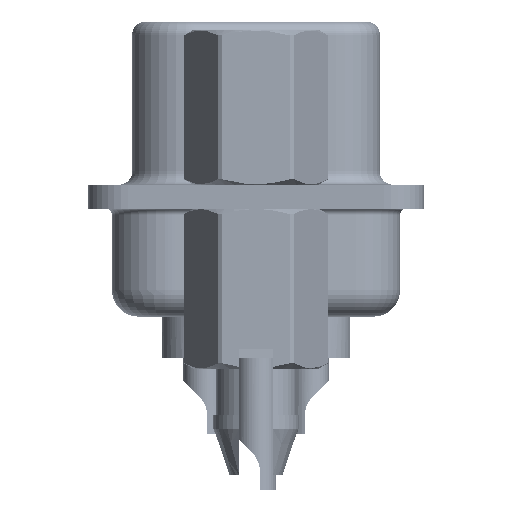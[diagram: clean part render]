
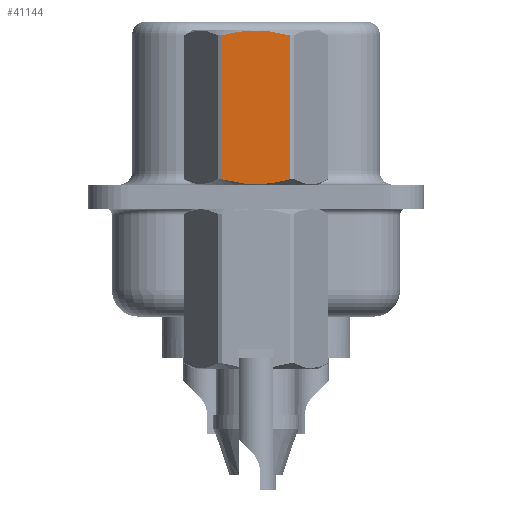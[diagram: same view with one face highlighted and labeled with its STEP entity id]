
A CAD part, left-side view. The second image highlights one B-rep face of the part: STEP entity #41144.
In plain terms, the highlighted planar face has unit normal (-1, 0, 0).
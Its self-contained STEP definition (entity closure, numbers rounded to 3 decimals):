
#478 = B_SPLINE_CURVE_WITH_KNOTS ( 'NONE', 3,
 ( #35614, #7081, #38136, #6877, #28891, #26176, #16082, #25345, #15880, #19857 ),
 .UNSPECIFIED., .F., .F.,
 ( 4, 2, 2, 2, 4 ),
 ( 0.003, 0.003, 0.004, 0.004, 0.005 ),
 .UNSPECIFIED. ) ;
#2210 = EDGE_CURVE ( 'NONE', #38166, #17996, #33887, .T. ) ;
#2494 = EDGE_CURVE ( 'NONE', #17996, #11123, #34546, .T. ) ;
#3700 = VECTOR ( 'NONE', #14819, 1000. ) ;
#4686 = DIRECTION ( 'NONE',  ( -1., 0., 0. ) ) ;
#5153 = DIRECTION ( 'NONE',  ( 0., 0., 1. ) ) ;
#6877 = CARTESIAN_POINT ( 'NONE',  ( -2.381, 0.428, 0.485 ) ) ;
#7081 = CARTESIAN_POINT ( 'NONE',  ( -2.381, 1.065, 0.596 ) ) ;
#8527 = VERTEX_POINT ( 'NONE', #16247 ) ;
#8683 = CARTESIAN_POINT ( 'NONE',  ( -2.381, -1.273, 6.048 ) ) ;
#10982 = PLANE ( 'NONE',  #33398 ) ;
#11123 = VERTEX_POINT ( 'NONE', #40946 ) ;
#12455 = CARTESIAN_POINT ( 'NONE',  ( -2.381, -1.066, 6.104 ) ) ;
#12660 = CARTESIAN_POINT ( 'NONE',  ( -2.381, -0.432, 6.215 ) ) ;
#13922 = CARTESIAN_POINT ( 'NONE',  ( -2.381, 1.375, -3.75 ) ) ;
#14133 = DIRECTION ( 'NONE',  ( 0., -1., 0. ) ) ;
#14336 = EDGE_CURVE ( 'NONE', #8527, #38166, #478, .T. ) ;
#14734 = FACE_OUTER_BOUND ( 'NONE', #26345, .T. ) ;
#14819 = DIRECTION ( 'NONE',  ( 0., 0., -1. ) ) ;
#15880 = CARTESIAN_POINT ( 'NONE',  ( -2.381, -1.066, 0.596 ) ) ;
#16082 = CARTESIAN_POINT ( 'NONE',  ( -2.381, -0.432, 0.485 ) ) ;
#16151 = VECTOR ( 'NONE', #5153, 1000. ) ;
#16247 = CARTESIAN_POINT ( 'NONE',  ( -2.381, 1.273, 0.652 ) ) ;
#17996 = VERTEX_POINT ( 'NONE', #21901 ) ;
#18160 = CARTESIAN_POINT ( 'NONE',  ( -2.381, -1.273, 3.792 ) ) ;
#19857 = CARTESIAN_POINT ( 'NONE',  ( -2.381, -1.273, 0.652 ) ) ;
#21158 = ORIENTED_EDGE ( 'NONE', *, *, #36408, .T. ) ;
#21901 = CARTESIAN_POINT ( 'NONE',  ( -2.381, -1.273, 6.048 ) ) ;
#21937 = CARTESIAN_POINT ( 'NONE',  ( -2.381, -1.273, 0.652 ) ) ;
#22112 = CARTESIAN_POINT ( 'NONE',  ( -2.381, 1.273, 6.048 ) ) ;
#23888 = LINE ( 'NONE', #24491, #3700 ) ;
#24491 = CARTESIAN_POINT ( 'NONE',  ( -2.381, 1.273, 3.792 ) ) ;
#25345 = CARTESIAN_POINT ( 'NONE',  ( -2.381, -0.858, 0.55 ) ) ;
#25475 = CARTESIAN_POINT ( 'NONE',  ( -2.381, -0.215, 6.232 ) ) ;
#26176 = CARTESIAN_POINT ( 'NONE',  ( -2.381, -0.215, 0.468 ) ) ;
#26345 = EDGE_LOOP ( 'NONE', ( #36290, #35183, #34044, #21158 ) ) ;
#28185 = CARTESIAN_POINT ( 'NONE',  ( -2.381, 0.853, 6.151 ) ) ;
#28610 = CARTESIAN_POINT ( 'NONE',  ( -2.381, 0.428, 6.215 ) ) ;
#28816 = CARTESIAN_POINT ( 'NONE',  ( -2.381, -0.858, 6.15 ) ) ;
#28891 = CARTESIAN_POINT ( 'NONE',  ( -2.381, 0.215, 0.468 ) ) ;
#33398 = AXIS2_PLACEMENT_3D ( 'NONE', #13922, #4686, #14133 ) ;
#33887 = LINE ( 'NONE', #18160, #16151 ) ;
#34044 = ORIENTED_EDGE ( 'NONE', *, *, #2494, .T. ) ;
#34546 = B_SPLINE_CURVE_WITH_KNOTS ( 'NONE', 3,
 ( #8683, #12455, #28816, #12660, #25475, #38056, #28610, #28185, #38261, #22112 ),
 .UNSPECIFIED., .F., .F.,
 ( 4, 2, 2, 2, 4 ),
 ( 0.001, 0.002, 0.002, 0.003, 0.004 ),
 .UNSPECIFIED. ) ;
#35183 = ORIENTED_EDGE ( 'NONE', *, *, #2210, .T. ) ;
#35614 = CARTESIAN_POINT ( 'NONE',  ( -2.381, 1.273, 0.652 ) ) ;
#36290 = ORIENTED_EDGE ( 'NONE', *, *, #14336, .T. ) ;
#36408 = EDGE_CURVE ( 'NONE', #11123, #8527, #23888, .T. ) ;
#38056 = CARTESIAN_POINT ( 'NONE',  ( -2.381, 0.215, 6.232 ) ) ;
#38136 = CARTESIAN_POINT ( 'NONE',  ( -2.381, 0.853, 0.549 ) ) ;
#38166 = VERTEX_POINT ( 'NONE', #21937 ) ;
#38261 = CARTESIAN_POINT ( 'NONE',  ( -2.381, 1.065, 6.104 ) ) ;
#40946 = CARTESIAN_POINT ( 'NONE',  ( -2.381, 1.273, 6.048 ) ) ;
#41144 = ADVANCED_FACE ( 'NONE', ( #14734 ), #10982, .T. ) ;
